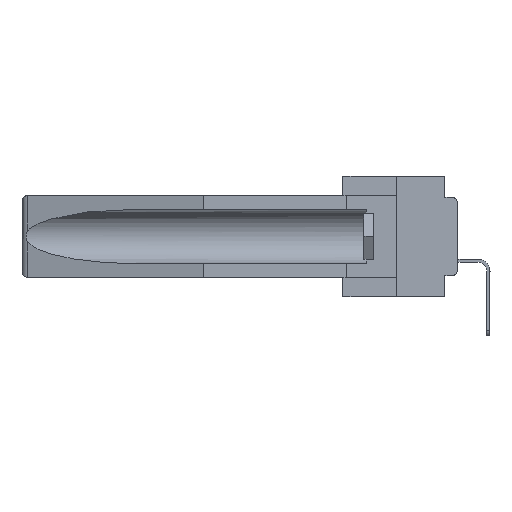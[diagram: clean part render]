
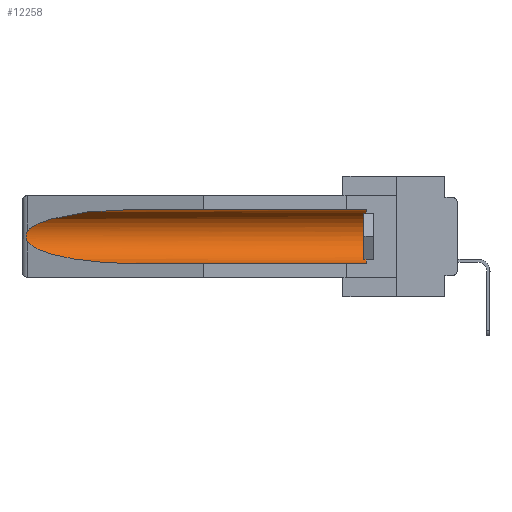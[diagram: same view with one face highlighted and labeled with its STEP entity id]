
A CAD part, left-side view. The second image highlights one B-rep face of the part: STEP entity #12258.
In plain terms, the highlighted cylindrical face has radius 2.857 mm (diameter 5.715 mm), a partial arc.
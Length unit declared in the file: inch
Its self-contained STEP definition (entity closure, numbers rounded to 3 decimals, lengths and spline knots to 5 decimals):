
#658 = CARTESIAN_POINT ( 'NONE',  ( 0.26537, 1.52718, -0.14972 ) ) ;
#2386 = DIRECTION ( 'NONE',  ( 0., 1., 0. ) ) ;
#2619 = CARTESIAN_POINT ( 'NONE',  ( 0.155, -0.30754, -0.059 ) ) ;
#2798 = CARTESIAN_POINT ( 'NONE',  ( 0.155, 0.126, -0.059 ) ) ;
#3384 = CARTESIAN_POINT ( 'NONE',  ( 0.21114, 1.30732, -0.284 ) ) ;
#3637 = CARTESIAN_POINT ( 'NONE',  ( 0.25451, 1.48313, -0.24835 ) ) ;
#3801 = CARTESIAN_POINT ( 'NONE',  ( 0.2673, 1.53269, -0.17917 ) ) ;
#3960 = AXIS2_PLACEMENT_3D ( 'NONE', #35949, #12630, #27275 ) ;
#5396 = DIRECTION ( 'NONE',  ( 0., 1., 0. ) ) ;
#5449 = AXIS2_PLACEMENT_3D ( 'NONE', #19679, #17252, #34575 ) ;
#5780 = B_SPLINE_CURVE_WITH_KNOTS ( 'NONE', 3,
 ( #658, #29953, #9668, #6866, #13128, #18488, #3801, #21665, #33263, #24470 ),
 .UNSPECIFIED., .F., .F.,
 ( 4, 2, 2, 2, 4 ),
 ( 0., 0.00029, 0.00058, 0.00087, 0.00117 ),
 .UNSPECIFIED. ) ;
#5970 = ORIENTED_EDGE ( 'NONE', *, *, #29352, .T. ) ;
#6399 = VECTOR ( 'NONE', #5396, 39.37008 ) ;
#6866 = CARTESIAN_POINT ( 'NONE',  ( 0.2673, 1.5327, -0.16383 ) ) ;
#7541 = VERTEX_POINT ( 'NONE', #13406 ) ;
#9668 = CARTESIAN_POINT ( 'NONE',  ( 0.26654, 1.53092, -0.15636 ) ) ;
#10984 = EDGE_CURVE ( 'NONE', #7541, #34850, #18889, .T. ) ;
#11393 = ORIENTED_EDGE ( 'NONE', *, *, #35673, .T. ) ;
#12258 = ADVANCED_FACE ( 'NONE', ( #17913 ), #22456, .F. ) ;
#12630 = DIRECTION ( 'NONE',  ( 0., -1., 0. ) ) ;
#13128 = CARTESIAN_POINT ( 'NONE',  ( 0.2675, 1.53308, -0.16763 ) ) ;
#13287 = EDGE_CURVE ( 'NONE', #15426, #15457, #26951, .T. ) ;
#13406 = CARTESIAN_POINT ( 'NONE',  ( 0.155, 1.07973, -0.059 ) ) ;
#15426 = VERTEX_POINT ( 'NONE', #34270 ) ;
#15457 = VERTEX_POINT ( 'NONE', #28517 ) ;
#15860 = ORIENTED_EDGE ( 'NONE', *, *, #26622, .T. ) ;
#16348 = ORIENTED_EDGE ( 'NONE', *, *, #10984, .T. ) ;
#16707 = CARTESIAN_POINT ( 'NONE',  ( 0.21114, 1.30732, -0.059 ) ) ;
#16923 = LINE ( 'NONE', #2619, #29677 ) ;
#17252 = DIRECTION ( 'NONE',  ( 0., 1., 0. ) ) ;
#17904 = ORIENTED_EDGE ( 'NONE', *, *, #26072, .T. ) ;
#17913 = FACE_OUTER_BOUND ( 'NONE', #21689, .T. ) ;
#18062 = CARTESIAN_POINT ( 'NONE',  ( 0.26537, 1.52718, -0.19328 ) ) ;
#18188 = ORIENTED_EDGE ( 'NONE', *, *, #13287, .F. ) ;
#18488 = CARTESIAN_POINT ( 'NONE',  ( 0.2675, 1.53308, -0.17534 ) ) ;
#18889 =( BOUNDED_CURVE ( )  B_SPLINE_CURVE ( 3, ( #34024, #16707, #37120, #19643 ),
 .UNSPECIFIED., .F., .F. ) 
 B_SPLINE_CURVE_WITH_KNOTS ( ( 4, 4 ),
 ( 4.71239, 6.08839 ),
 .UNSPECIFIED. ) 
 CURVE ( )  GEOMETRIC_REPRESENTATION_ITEM ( )  RATIONAL_B_SPLINE_CURVE ( ( 1., 0.848, 0.848, 1. ) ) 
 REPRESENTATION_ITEM ( '' )  );
#19643 = CARTESIAN_POINT ( 'NONE',  ( 0.26537, 1.52718, -0.14972 ) ) ;
#19679 = CARTESIAN_POINT ( 'NONE',  ( 0.155, -0.30754, -0.1715 ) ) ;
#20323 = CARTESIAN_POINT ( 'NONE',  ( 0.155, -0.30754, -0.284 ) ) ;
#21665 = CARTESIAN_POINT ( 'NONE',  ( 0.26655, 1.53094, -0.18657 ) ) ;
#21689 = EDGE_LOOP ( 'NONE', ( #16348, #17904, #15860, #18188, #11393, #5970 ) ) ;
#22456 = CYLINDRICAL_SURFACE ( 'NONE', #5449, 0.1125 ) ;
#23633 = CARTESIAN_POINT ( 'NONE',  ( 0.26537, 1.52718, -0.14972 ) ) ;
#24470 = CARTESIAN_POINT ( 'NONE',  ( 0.26537, 1.52718, -0.19328 ) ) ;
#25874 = VERTEX_POINT ( 'NONE', #2798 ) ;
#26072 = EDGE_CURVE ( 'NONE', #34850, #31922, #5780, .T. ) ;
#26622 = EDGE_CURVE ( 'NONE', #31922, #15457, #28921, .T. ) ;
#26869 = CARTESIAN_POINT ( 'NONE',  ( 0.155, 1.07973, -0.284 ) ) ;
#26951 = LINE ( 'NONE', #20323, #6399 ) ;
#27275 = DIRECTION ( 'NONE',  ( 0., 0., 1. ) ) ;
#28517 = CARTESIAN_POINT ( 'NONE',  ( 0.155, 1.07973, -0.284 ) ) ;
#28921 =( BOUNDED_CURVE ( )  B_SPLINE_CURVE ( 3, ( #18062, #3637, #3384, #26869 ),
 .UNSPECIFIED., .F., .F. ) 
 B_SPLINE_CURVE_WITH_KNOTS ( ( 4, 4 ),
 ( 0.1948, 1.5708 ),
 .UNSPECIFIED. ) 
 CURVE ( )  GEOMETRIC_REPRESENTATION_ITEM ( )  RATIONAL_B_SPLINE_CURVE ( ( 1., 0.848, 0.848, 1. ) ) 
 REPRESENTATION_ITEM ( '' )  );
#29352 = EDGE_CURVE ( 'NONE', #25874, #7541, #16923, .T. ) ;
#29677 = VECTOR ( 'NONE', #2386, 39.37008 ) ;
#29953 = CARTESIAN_POINT ( 'NONE',  ( 0.26597, 1.52961, -0.15275 ) ) ;
#30545 = CARTESIAN_POINT ( 'NONE',  ( 0.26537, 1.52718, -0.19328 ) ) ;
#31922 = VERTEX_POINT ( 'NONE', #30545 ) ;
#33263 = CARTESIAN_POINT ( 'NONE',  ( 0.26597, 1.5296, -0.19026 ) ) ;
#34024 = CARTESIAN_POINT ( 'NONE',  ( 0.155, 1.07973, -0.059 ) ) ;
#34270 = CARTESIAN_POINT ( 'NONE',  ( 0.155, 0.126, -0.284 ) ) ;
#34575 = DIRECTION ( 'NONE',  ( 0., 0., 1. ) ) ;
#34850 = VERTEX_POINT ( 'NONE', #23633 ) ;
#35056 = CIRCLE ( 'NONE', #3960, 0.1125 ) ;
#35673 = EDGE_CURVE ( 'NONE', #15426, #25874, #35056, .T. ) ;
#35949 = CARTESIAN_POINT ( 'NONE',  ( 0.155, 0.126, -0.1715 ) ) ;
#37120 = CARTESIAN_POINT ( 'NONE',  ( 0.25451, 1.48313, -0.09465 ) ) ;
